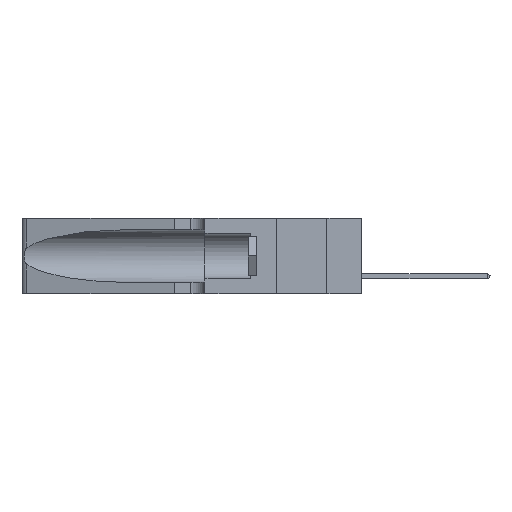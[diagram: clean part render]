
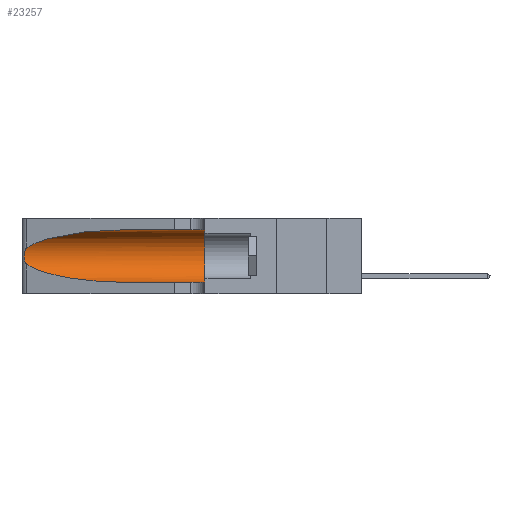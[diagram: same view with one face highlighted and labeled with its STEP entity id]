
A CAD part, left-side view. The second image highlights one B-rep face of the part: STEP entity #23257.
In plain terms, the highlighted cylindrical face has radius 3.308 mm (diameter 6.617 mm), a partial arc.
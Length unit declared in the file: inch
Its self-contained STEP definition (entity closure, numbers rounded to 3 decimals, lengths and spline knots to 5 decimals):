
#73 = B_SPLINE_CURVE_WITH_KNOTS ( 'NONE', 3,
 ( #19424, #6308, #10450, #38987, #46382, #35821, #39455, #6639, #17750, #43073, #13800, #21357, #46061, #13645 ),
 .UNSPECIFIED., .F., .F.,
 ( 4, 2, 2, 2, 2, 2, 4 ),
 ( 0., 0.00027, 0.00053, 0.00107, 0.0016, 0.00187, 0.00214 ),
 .UNSPECIFIED. ) ;
#1704 = CYLINDRICAL_SURFACE ( 'NONE', #29247, 0.13025 ) ;
#2039 = CARTESIAN_POINT ( 'NONE',  ( 0.25487, 1.22718, 0.22369 ) ) ;
#4340 = CARTESIAN_POINT ( 'NONE',  ( 0.1305, 0.35, 0.31525 ) ) ;
#6034 = EDGE_CURVE ( 'NONE', #39085, #37843, #38637, .T. ) ;
#6308 = CARTESIAN_POINT ( 'NONE',  ( 0.25555, 1.22994, 0.2215 ) ) ;
#6639 = CARTESIAN_POINT ( 'NONE',  ( 0.26075, 1.23896, 0.178 ) ) ;
#8892 = CARTESIAN_POINT ( 'NONE',  ( 0.18966, 0.96281, 0.31525 ) ) ;
#10402 = ORIENTED_EDGE ( 'NONE', *, *, #6034, .F. ) ;
#10450 = CARTESIAN_POINT ( 'NONE',  ( 0.25639, 1.23184, 0.21858 ) ) ;
#10730 = VERTEX_POINT ( 'NONE', #29150 ) ;
#11376 =( BOUNDED_CURVE ( )  B_SPLINE_CURVE ( 3, ( #30464, #8892, #19793, #2039 ),
 .UNSPECIFIED., .F., .T. ) 
 B_SPLINE_CURVE_WITH_KNOTS ( ( 4, 4 ),
 ( 1.5708, 2.84003 ),
 .UNSPECIFIED. ) 
 CURVE ( )  GEOMETRIC_REPRESENTATION_ITEM ( )  RATIONAL_B_SPLINE_CURVE ( ( 1., 0.87, 0.87, 1. ) ) 
 REPRESENTATION_ITEM ( '' )  );
#11652 = VERTEX_POINT ( 'NONE', #19330 ) ;
#11967 = EDGE_CURVE ( 'NONE', #11652, #10730, #19751, .T. ) ;
#12920 = DIRECTION ( 'NONE',  ( 0., -1., 0. ) ) ;
#12924 = LINE ( 'NONE', #21136, #42975 ) ;
#13383 = CARTESIAN_POINT ( 'NONE',  ( 0.25487, 1.22718, 0.22369 ) ) ;
#13645 = CARTESIAN_POINT ( 'NONE',  ( 0.25487, 1.22718, 0.14631 ) ) ;
#13800 = CARTESIAN_POINT ( 'NONE',  ( 0.25789, 1.23486, 0.15765 ) ) ;
#15391 = ORIENTED_EDGE ( 'NONE', *, *, #17687, .T. ) ;
#15541 = ORIENTED_EDGE ( 'NONE', *, *, #29509, .T. ) ;
#15602 = CARTESIAN_POINT ( 'NONE',  ( 0.25487, 1.22718, 0.14631 ) ) ;
#17687 = EDGE_CURVE ( 'NONE', #10730, #37843, #12924, .T. ) ;
#17750 = CARTESIAN_POINT ( 'NONE',  ( 0.26017, 1.23833, 0.17102 ) ) ;
#19330 = CARTESIAN_POINT ( 'NONE',  ( 0.25487, 1.22718, 0.14631 ) ) ;
#19424 = CARTESIAN_POINT ( 'NONE',  ( 0.25487, 1.22718, 0.22369 ) ) ;
#19665 = CARTESIAN_POINT ( 'NONE',  ( 0.1305, 0.35, 0.05475 ) ) ;
#19751 =( BOUNDED_CURVE ( )  B_SPLINE_CURVE ( 3, ( #15602, #34280, #20912, #28229 ),
 .UNSPECIFIED., .F., .T. ) 
 B_SPLINE_CURVE_WITH_KNOTS ( ( 4, 4 ),
 ( 3.44316, 4.71239 ),
 .UNSPECIFIED. ) 
 CURVE ( )  GEOMETRIC_REPRESENTATION_ITEM ( )  RATIONAL_B_SPLINE_CURVE ( ( 1., 0.87, 0.87, 1. ) ) 
 REPRESENTATION_ITEM ( '' )  );
#19793 = CARTESIAN_POINT ( 'NONE',  ( 0.2373, 1.15595, 0.28018 ) ) ;
#20912 = CARTESIAN_POINT ( 'NONE',  ( 0.18966, 0.96281, 0.05475 ) ) ;
#21136 = CARTESIAN_POINT ( 'NONE',  ( 0.1305, 1.61858, 0.05475 ) ) ;
#21357 = CARTESIAN_POINT ( 'NONE',  ( 0.25639, 1.23186, 0.15144 ) ) ;
#21553 = ORIENTED_EDGE ( 'NONE', *, *, #28474, .T. ) ;
#22512 = AXIS2_PLACEMENT_3D ( 'NONE', #44390, #38427, #23320 ) ;
#23257 = ADVANCED_FACE ( 'NONE', ( #38685 ), #1704, .F. ) ;
#23320 = DIRECTION ( 'NONE',  ( 0., 0., 1. ) ) ;
#23372 = VECTOR ( 'NONE', #30189, 39.37008 ) ;
#25313 = EDGE_LOOP ( 'NONE', ( #21553, #15541, #42559, #15391, #10402, #42648 ) ) ;
#27120 = VERTEX_POINT ( 'NONE', #13383 ) ;
#28229 = CARTESIAN_POINT ( 'NONE',  ( 0.1305, 0.72297, 0.05475 ) ) ;
#28474 = EDGE_CURVE ( 'NONE', #34907, #27120, #11376, .T. ) ;
#29150 = CARTESIAN_POINT ( 'NONE',  ( 0.1305, 0.72297, 0.05475 ) ) ;
#29247 = AXIS2_PLACEMENT_3D ( 'NONE', #30979, #12920, #41888 ) ;
#29509 = EDGE_CURVE ( 'NONE', #27120, #11652, #73, .T. ) ;
#30189 = DIRECTION ( 'NONE',  ( 0., -1., 0. ) ) ;
#30464 = CARTESIAN_POINT ( 'NONE',  ( 0.1305, 0.72297, 0.31525 ) ) ;
#30979 = CARTESIAN_POINT ( 'NONE',  ( 0.1305, 1.61858, 0.185 ) ) ;
#33656 = CARTESIAN_POINT ( 'NONE',  ( 0.1305, 1.61858, 0.31525 ) ) ;
#34188 = LINE ( 'NONE', #33656, #23372 ) ;
#34280 = CARTESIAN_POINT ( 'NONE',  ( 0.2373, 1.15595, 0.08982 ) ) ;
#34907 = VERTEX_POINT ( 'NONE', #45158 ) ;
#35821 = CARTESIAN_POINT ( 'NONE',  ( 0.26018, 1.23835, 0.19895 ) ) ;
#37843 = VERTEX_POINT ( 'NONE', #19665 ) ;
#38427 = DIRECTION ( 'NONE',  ( 0., 1., 0. ) ) ;
#38637 = CIRCLE ( 'NONE', #22512, 0.13025 ) ;
#38685 = FACE_OUTER_BOUND ( 'NONE', #25313, .T. ) ;
#38987 = CARTESIAN_POINT ( 'NONE',  ( 0.25787, 1.23484, 0.2124 ) ) ;
#39085 = VERTEX_POINT ( 'NONE', #4340 ) ;
#39455 = CARTESIAN_POINT ( 'NONE',  ( 0.26075, 1.23896, 0.19203 ) ) ;
#41888 = DIRECTION ( 'NONE',  ( 0., 0., -1. ) ) ;
#42559 = ORIENTED_EDGE ( 'NONE', *, *, #11967, .T. ) ;
#42648 = ORIENTED_EDGE ( 'NONE', *, *, #45304, .F. ) ;
#42975 = VECTOR ( 'NONE', #46785, 39.37008 ) ;
#43073 = CARTESIAN_POINT ( 'NONE',  ( 0.25856, 1.23593, 0.16098 ) ) ;
#44390 = CARTESIAN_POINT ( 'NONE',  ( 0.1305, 0.35, 0.185 ) ) ;
#45158 = CARTESIAN_POINT ( 'NONE',  ( 0.1305, 0.72297, 0.31525 ) ) ;
#45304 = EDGE_CURVE ( 'NONE', #34907, #39085, #34188, .T. ) ;
#46061 = CARTESIAN_POINT ( 'NONE',  ( 0.25555, 1.22993, 0.14849 ) ) ;
#46382 = CARTESIAN_POINT ( 'NONE',  ( 0.25854, 1.2359, 0.20912 ) ) ;
#46785 = DIRECTION ( 'NONE',  ( 0., -1., 0. ) ) ;
